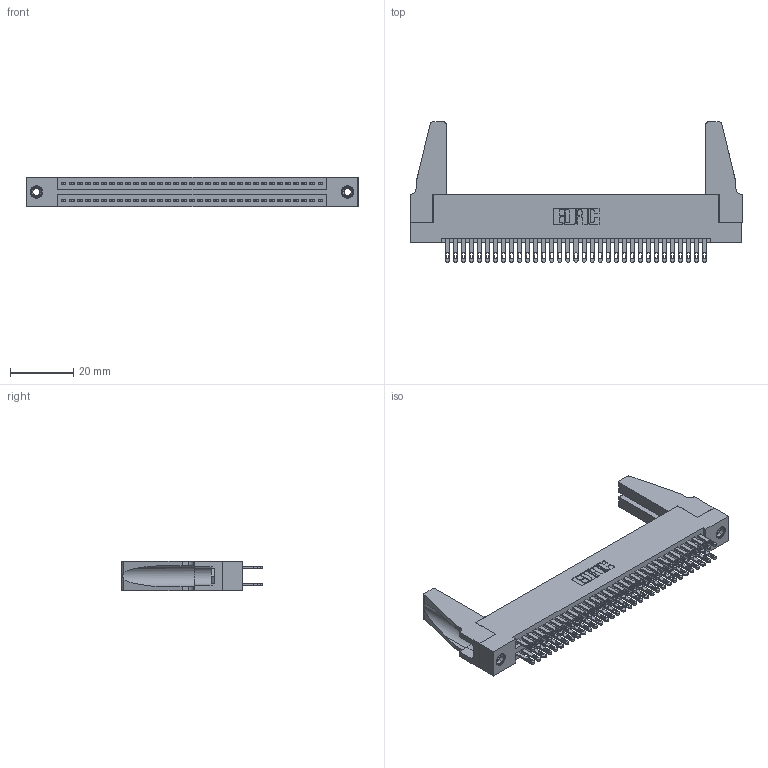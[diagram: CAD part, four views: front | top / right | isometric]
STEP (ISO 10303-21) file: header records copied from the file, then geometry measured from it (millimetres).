
FILE_DESCRIPTION (( 'STEP AP203' ), '1' );
FILE_NAME ('345-066-500-288.STEP', '2019-10-30T15:51:21', ( '' ), ( '' ), 'SwSTEP 2.0', 'SolidWorks 2016', '' );
FILE_SCHEMA (( 'CONFIG_CONTROL_DESIGN' ));
Length unit declared in the file: inch
Products named in the file (5): 345-066-500-288; 345-220-078_345-220-088; 345-292-001_345-293-100; 345-250-001_345-250-001-102; 345 Part_Flush Mounting Lugs - 0.156 Dia-TH
Assembly tree (71 placements, depth 2):
  345-066-500-288
    345 Part_Flush Mounting Lugs - 0.156 Dia-TH
    345-292-001_345-293-100  x66
    345-250-001_345-250-001-102  x2
    345-220-078_345-220-088  x2
Bounding box: 105.05 x 44.37 x 9.4 mm (x, y, z)
Volume: 13575.7 mm3; surface area: 18880.5 mm2
Topology: 71 solids, 71 shells, 3286 faces, 9961 edges, 6630 vertices
Faces by surface type: plane 1934, cylinder 1336, cone 12, torus 4
Entity records: 29182 total; most frequent: CARTESIAN_POINT 4894, ORIENTED_EDGE 4788, DIRECTION 4334, EDGE_CURVE 2394, LINE 2084, VECTOR 2084, VERTEX_POINT 1590, AXIS2_PLACEMENT_3D 1125
